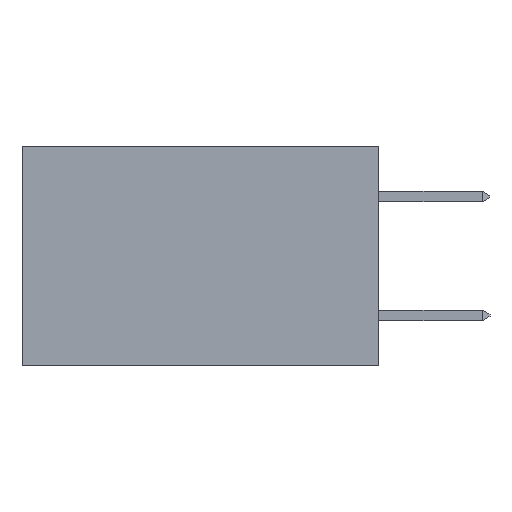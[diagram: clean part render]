
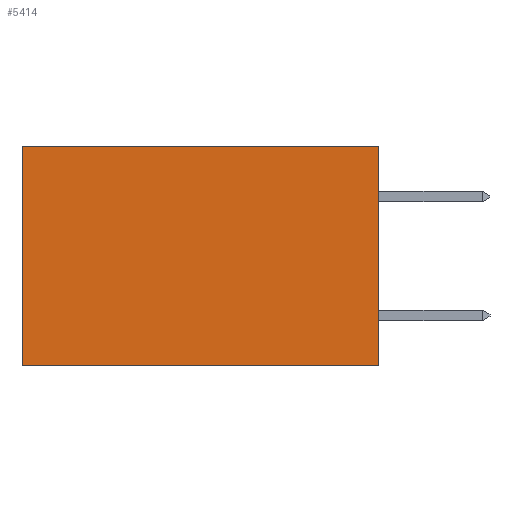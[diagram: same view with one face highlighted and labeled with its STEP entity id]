
A CAD part, left-side view. The second image highlights one B-rep face of the part: STEP entity #5414.
In plain terms, the highlighted planar face has unit normal (-1, 0, 0).
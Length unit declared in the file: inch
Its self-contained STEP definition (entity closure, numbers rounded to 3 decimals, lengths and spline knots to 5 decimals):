
#451 = AXIS2_PLACEMENT_3D ( 'NONE', #8922, #5347, #971 ) ;
#765 = LINE ( 'NONE', #3104, #4436 ) ;
#971 = DIRECTION ( 'NONE',  ( 0., 0., -1. ) ) ;
#1139 = LINE ( 'NONE', #1159, #4797 ) ;
#1159 = CARTESIAN_POINT ( 'NONE',  ( 0.2615, 0., 0. ) ) ;
#1765 = CARTESIAN_POINT ( 'NONE',  ( 0.2615, 0., -0.37 ) ) ;
#1924 = LINE ( 'NONE', #4397, #9361 ) ;
#1935 = EDGE_CURVE ( 'NONE', #4488, #3732, #1139, .T. ) ;
#2156 = VERTEX_POINT ( 'NONE', #1765 ) ;
#2221 = DIRECTION ( 'NONE',  ( 0., 1., 0. ) ) ;
#2346 = VECTOR ( 'NONE', #4850, 39.37008 ) ;
#2673 = EDGE_CURVE ( 'NONE', #4488, #2156, #765, .T. ) ;
#2695 = ORIENTED_EDGE ( 'NONE', *, *, #5628, .T. ) ;
#2913 = CARTESIAN_POINT ( 'NONE',  ( 0.2615, 0., 0. ) ) ;
#3059 = DIRECTION ( 'NONE',  ( 0., 0., -1. ) ) ;
#3104 = CARTESIAN_POINT ( 'NONE',  ( 0.2615, 0., -0.37 ) ) ;
#3402 = EDGE_CURVE ( 'NONE', #2156, #8565, #1924, .T. ) ;
#3732 = VERTEX_POINT ( 'NONE', #8440 ) ;
#4248 = ORIENTED_EDGE ( 'NONE', *, *, #1935, .T. ) ;
#4397 = CARTESIAN_POINT ( 'NONE',  ( 0.2615, 0., -0.37 ) ) ;
#4436 = VECTOR ( 'NONE', #3059, 39.37008 ) ;
#4488 = VERTEX_POINT ( 'NONE', #2913 ) ;
#4797 = VECTOR ( 'NONE', #2221, 39.37008 ) ;
#4850 = DIRECTION ( 'NONE',  ( 0., 0., -1. ) ) ;
#5347 = DIRECTION ( 'NONE',  ( 1., 0., 0. ) ) ;
#5382 = ORIENTED_EDGE ( 'NONE', *, *, #3402, .F. ) ;
#5414 = ADVANCED_FACE ( 'NONE', ( #7656 ), #6034, .F. ) ;
#5628 = EDGE_CURVE ( 'NONE', #3732, #8565, #6176, .T. ) ;
#6034 = PLANE ( 'NONE',  #451 ) ;
#6176 = LINE ( 'NONE', #9143, #2346 ) ;
#6582 = DIRECTION ( 'NONE',  ( 0., 1., 0. ) ) ;
#6676 = ORIENTED_EDGE ( 'NONE', *, *, #2673, .F. ) ;
#7043 = EDGE_LOOP ( 'NONE', ( #2695, #5382, #6676, #4248 ) ) ;
#7656 = FACE_OUTER_BOUND ( 'NONE', #7043, .T. ) ;
#8440 = CARTESIAN_POINT ( 'NONE',  ( 0.2615, 0.6, 0. ) ) ;
#8565 = VERTEX_POINT ( 'NONE', #8783 ) ;
#8783 = CARTESIAN_POINT ( 'NONE',  ( 0.2615, 0.6, -0.37 ) ) ;
#8922 = CARTESIAN_POINT ( 'NONE',  ( 0.2615, 0., -0.37 ) ) ;
#9143 = CARTESIAN_POINT ( 'NONE',  ( 0.2615, 0.6, -0.37 ) ) ;
#9361 = VECTOR ( 'NONE', #6582, 39.37008 ) ;
